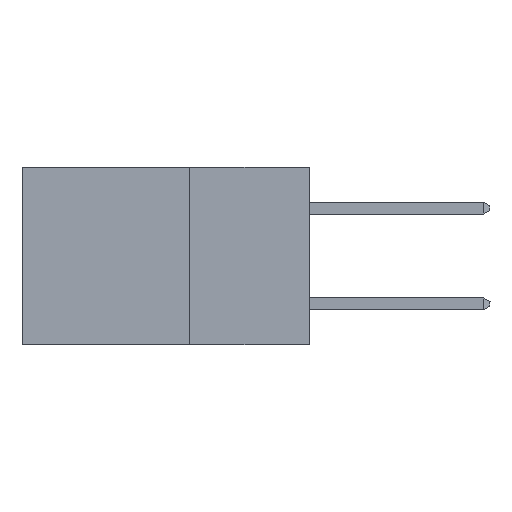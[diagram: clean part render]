
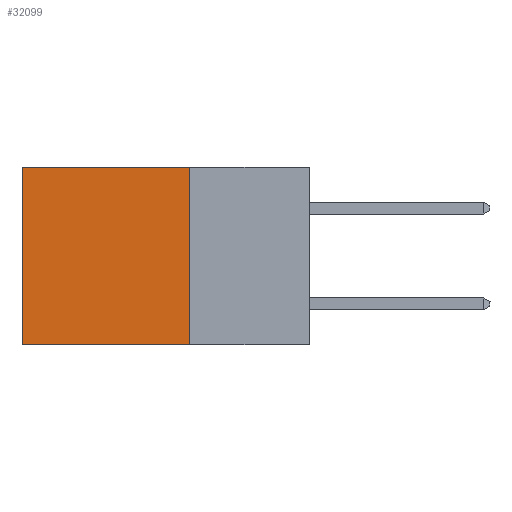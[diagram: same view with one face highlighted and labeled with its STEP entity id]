
A CAD part, left-side view. The second image highlights one B-rep face of the part: STEP entity #32099.
In plain terms, the highlighted planar face has unit normal (-1, 0, 0).
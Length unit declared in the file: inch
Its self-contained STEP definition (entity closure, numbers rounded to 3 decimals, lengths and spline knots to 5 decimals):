
#1437 = DIRECTION ( 'NONE',  ( 0., 0., -1. ) ) ;
#3690 = LINE ( 'NONE', #11467, #30088 ) ;
#4849 = ORIENTED_EDGE ( 'NONE', *, *, #36498, .T. ) ;
#7681 = VECTOR ( 'NONE', #37139, 39.37008 ) ;
#8140 = VECTOR ( 'NONE', #8837, 39.37008 ) ;
#8837 = DIRECTION ( 'NONE',  ( 0., 1., 0. ) ) ;
#11467 = CARTESIAN_POINT ( 'NONE',  ( 0.2875, 0.6, 0. ) ) ;
#13169 = EDGE_CURVE ( 'NONE', #40725, #43465, #33116, .T. ) ;
#13569 = LINE ( 'NONE', #25725, #8140 ) ;
#14614 = EDGE_CURVE ( 'NONE', #40725, #34070, #13569, .T. ) ;
#15029 = PLANE ( 'NONE',  #16278 ) ;
#15839 = LINE ( 'NONE', #26893, #7681 ) ;
#16278 = AXIS2_PLACEMENT_3D ( 'NONE', #28855, #21981, #35664 ) ;
#18997 = EDGE_LOOP ( 'NONE', ( #4849, #22720, #22914, #22894 ) ) ;
#20255 = FACE_OUTER_BOUND ( 'NONE', #18997, .T. ) ;
#20992 = VERTEX_POINT ( 'NONE', #35976 ) ;
#21595 = DIRECTION ( 'NONE',  ( 0., 0., -1. ) ) ;
#21981 = DIRECTION ( 'NONE',  ( 1., 0., 0. ) ) ;
#22720 = ORIENTED_EDGE ( 'NONE', *, *, #33484, .F. ) ;
#22894 = ORIENTED_EDGE ( 'NONE', *, *, #14614, .T. ) ;
#22914 = ORIENTED_EDGE ( 'NONE', *, *, #13169, .F. ) ;
#25725 = CARTESIAN_POINT ( 'NONE',  ( 0.2875, 0.25, 0. ) ) ;
#26893 = CARTESIAN_POINT ( 'NONE',  ( 0.2875, 0.25, -0.37 ) ) ;
#28855 = CARTESIAN_POINT ( 'NONE',  ( 0.2875, 0.25, 0. ) ) ;
#30088 = VECTOR ( 'NONE', #21595, 39.37008 ) ;
#31838 = CARTESIAN_POINT ( 'NONE',  ( 0.2875, 0.25, 0. ) ) ;
#32099 = ADVANCED_FACE ( 'NONE', ( #20255 ), #15029, .F. ) ;
#33116 = LINE ( 'NONE', #31838, #33651 ) ;
#33212 = CARTESIAN_POINT ( 'NONE',  ( 0.2875, 0.6, 0. ) ) ;
#33484 = EDGE_CURVE ( 'NONE', #43465, #20992, #15839, .T. ) ;
#33651 = VECTOR ( 'NONE', #1437, 39.37008 ) ;
#34070 = VERTEX_POINT ( 'NONE', #33212 ) ;
#35664 = DIRECTION ( 'NONE',  ( 0., 0., -1. ) ) ;
#35976 = CARTESIAN_POINT ( 'NONE',  ( 0.2875, 0.6, -0.37 ) ) ;
#36498 = EDGE_CURVE ( 'NONE', #34070, #20992, #3690, .T. ) ;
#37139 = DIRECTION ( 'NONE',  ( 0., 1., 0. ) ) ;
#40725 = VERTEX_POINT ( 'NONE', #40875 ) ;
#40875 = CARTESIAN_POINT ( 'NONE',  ( 0.2875, 0.25, 0. ) ) ;
#43465 = VERTEX_POINT ( 'NONE', #43963 ) ;
#43963 = CARTESIAN_POINT ( 'NONE',  ( 0.2875, 0.25, -0.37 ) ) ;
